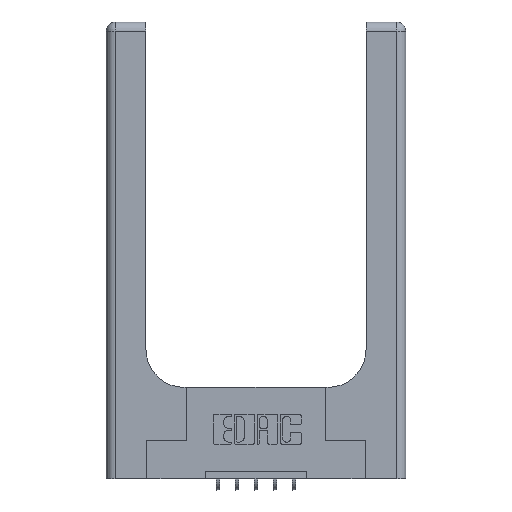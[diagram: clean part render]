
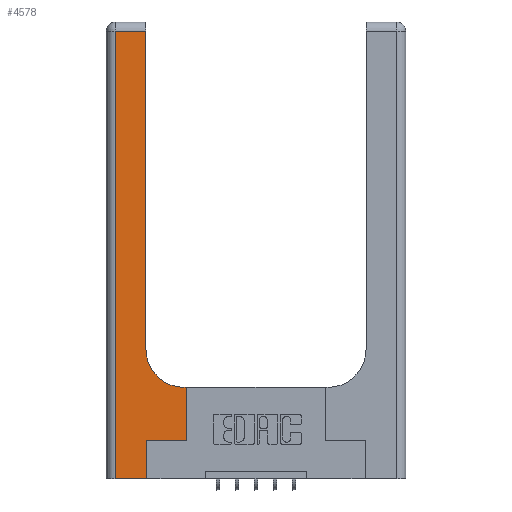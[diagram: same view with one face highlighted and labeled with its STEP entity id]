
A CAD part, top view. The second image highlights one B-rep face of the part: STEP entity #4578.
In plain terms, the highlighted planar face has unit normal (0, 0, 1).
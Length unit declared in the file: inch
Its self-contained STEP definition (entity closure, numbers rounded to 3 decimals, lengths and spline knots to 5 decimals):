
#33 = CARTESIAN_POINT ( 'NONE',  ( 0.528, 0.25, 0.37 ) ) ;
#72 = CARTESIAN_POINT ( 'NONE',  ( 0.06, 0., 0.37 ) ) ;
#448 = EDGE_CURVE ( 'NONE', #958, #7667, #4107, .T. ) ;
#598 = ORIENTED_EDGE ( 'NONE', *, *, #13527, .T. ) ;
#958 = VERTEX_POINT ( 'NONE', #6147 ) ;
#1785 = CARTESIAN_POINT ( 'NONE',  ( 0., 2.94, 0.37 ) ) ;
#1970 = DIRECTION ( 'NONE',  ( 0., 1., 0. ) ) ;
#2192 = DIRECTION ( 'NONE',  ( 0., 0., -1. ) ) ;
#2345 = VERTEX_POINT ( 'NONE', #7071 ) ;
#2385 = CARTESIAN_POINT ( 'NONE',  ( 0.26, 3., 0.37 ) ) ;
#2583 = EDGE_CURVE ( 'NONE', #4966, #5000, #3834, .T. ) ;
#2949 = VERTEX_POINT ( 'NONE', #72 ) ;
#3742 = EDGE_CURVE ( 'NONE', #4122, #2345, #13313, .T. ) ;
#3748 = VECTOR ( 'NONE', #5990, 39.37008 ) ;
#3834 = LINE ( 'NONE', #13319, #5085 ) ;
#4107 = LINE ( 'NONE', #11631, #11542 ) ;
#4122 = VERTEX_POINT ( 'NONE', #6446 ) ;
#4209 = PLANE ( 'NONE',  #6332 ) ;
#4450 = VECTOR ( 'NONE', #1970, 39.37008 ) ;
#4578 = ADVANCED_FACE ( 'NONE', ( #11511 ), #4209, .F. ) ;
#4966 = VERTEX_POINT ( 'NONE', #6770 ) ;
#4991 = ORIENTED_EDGE ( 'NONE', *, *, #11961, .T. ) ;
#5000 = VERTEX_POINT ( 'NONE', #5560 ) ;
#5085 = VECTOR ( 'NONE', #9078, 39.37008 ) ;
#5268 = VECTOR ( 'NONE', #7500, 39.37008 ) ;
#5560 = CARTESIAN_POINT ( 'NONE',  ( 0.51, 0.6, 0.37 ) ) ;
#5990 = DIRECTION ( 'NONE',  ( -1., 0., 0. ) ) ;
#6095 = LINE ( 'NONE', #10264, #12066 ) ;
#6130 = DIRECTION ( 'NONE',  ( 0., 1., 0. ) ) ;
#6147 = CARTESIAN_POINT ( 'NONE',  ( 0.265, 0., 0.37 ) ) ;
#6151 = VERTEX_POINT ( 'NONE', #12950 ) ;
#6169 = EDGE_CURVE ( 'NONE', #6151, #4122, #12039, .T. ) ;
#6285 = DIRECTION ( 'NONE',  ( -1., 0., 0. ) ) ;
#6332 = AXIS2_PLACEMENT_3D ( 'NONE', #12835, #2192, #6285 ) ;
#6401 = AXIS2_PLACEMENT_3D ( 'NONE', #10769, #9562, #10543 ) ;
#6446 = CARTESIAN_POINT ( 'NONE',  ( 0.26, 2.94, 0.37 ) ) ;
#6770 = CARTESIAN_POINT ( 'NONE',  ( 0.528, 0.6, 0.37 ) ) ;
#7071 = CARTESIAN_POINT ( 'NONE',  ( 0.06, 2.94, 0.37 ) ) ;
#7500 = DIRECTION ( 'NONE',  ( 1., 0., 0. ) ) ;
#7667 = VERTEX_POINT ( 'NONE', #13744 ) ;
#8338 = LINE ( 'NONE', #12937, #5268 ) ;
#8664 = ORIENTED_EDGE ( 'NONE', *, *, #10985, .T. ) ;
#8694 = VERTEX_POINT ( 'NONE', #33 ) ;
#8940 = VECTOR ( 'NONE', #13013, 39.37008 ) ;
#9078 = DIRECTION ( 'NONE',  ( -1., 0., 0. ) ) ;
#9270 = LINE ( 'NONE', #9337, #9866 ) ;
#9337 = CARTESIAN_POINT ( 'NONE',  ( 0.06, 3., 0.37 ) ) ;
#9562 = DIRECTION ( 'NONE',  ( 0., 0., -1. ) ) ;
#9866 = VECTOR ( 'NONE', #13492, 39.37008 ) ;
#10030 = ORIENTED_EDGE ( 'NONE', *, *, #3742, .T. ) ;
#10122 = EDGE_LOOP ( 'NONE', ( #12562, #10030, #11709, #13654, #11844, #4991, #598, #11558, #8664 ) ) ;
#10264 = CARTESIAN_POINT ( 'NONE',  ( 0.265, 0.25, 0.37 ) ) ;
#10543 = DIRECTION ( 'NONE',  ( 1., 0., 0. ) ) ;
#10565 = EDGE_CURVE ( 'NONE', #2949, #958, #8338, .T. ) ;
#10566 = CARTESIAN_POINT ( 'NONE',  ( 0.528, 0.25, 0.37 ) ) ;
#10769 = CARTESIAN_POINT ( 'NONE',  ( 0.51, 0.85, 0.37 ) ) ;
#10985 = EDGE_CURVE ( 'NONE', #5000, #6151, #12067, .T. ) ;
#11479 = LINE ( 'NONE', #10566, #4450 ) ;
#11511 = FACE_OUTER_BOUND ( 'NONE', #10122, .T. ) ;
#11542 = VECTOR ( 'NONE', #6130, 39.37008 ) ;
#11558 = ORIENTED_EDGE ( 'NONE', *, *, #2583, .T. ) ;
#11631 = CARTESIAN_POINT ( 'NONE',  ( 0.265, 0., 0.37 ) ) ;
#11709 = ORIENTED_EDGE ( 'NONE', *, *, #13703, .T. ) ;
#11844 = ORIENTED_EDGE ( 'NONE', *, *, #448, .T. ) ;
#11961 = EDGE_CURVE ( 'NONE', #7667, #8694, #6095, .T. ) ;
#12039 = LINE ( 'NONE', #2385, #8940 ) ;
#12066 = VECTOR ( 'NONE', #12431, 39.37008 ) ;
#12067 = CIRCLE ( 'NONE', #6401, 0.25 ) ;
#12431 = DIRECTION ( 'NONE',  ( 1., 0., 0. ) ) ;
#12562 = ORIENTED_EDGE ( 'NONE', *, *, #6169, .T. ) ;
#12835 = CARTESIAN_POINT ( 'NONE',  ( 0., 3., 0.37 ) ) ;
#12937 = CARTESIAN_POINT ( 'NONE',  ( 0., 0., 0.37 ) ) ;
#12950 = CARTESIAN_POINT ( 'NONE',  ( 0.26, 0.85, 0.37 ) ) ;
#13013 = DIRECTION ( 'NONE',  ( 0., 1., 0. ) ) ;
#13313 = LINE ( 'NONE', #1785, #3748 ) ;
#13319 = CARTESIAN_POINT ( 'NONE',  ( 0.26, 0.6, 0.37 ) ) ;
#13492 = DIRECTION ( 'NONE',  ( 0., -1., 0. ) ) ;
#13527 = EDGE_CURVE ( 'NONE', #8694, #4966, #11479, .T. ) ;
#13654 = ORIENTED_EDGE ( 'NONE', *, *, #10565, .T. ) ;
#13703 = EDGE_CURVE ( 'NONE', #2345, #2949, #9270, .T. ) ;
#13744 = CARTESIAN_POINT ( 'NONE',  ( 0.265, 0.25, 0.37 ) ) ;
